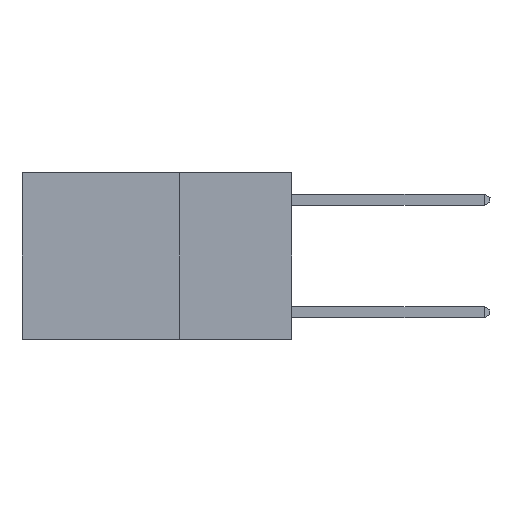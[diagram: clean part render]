
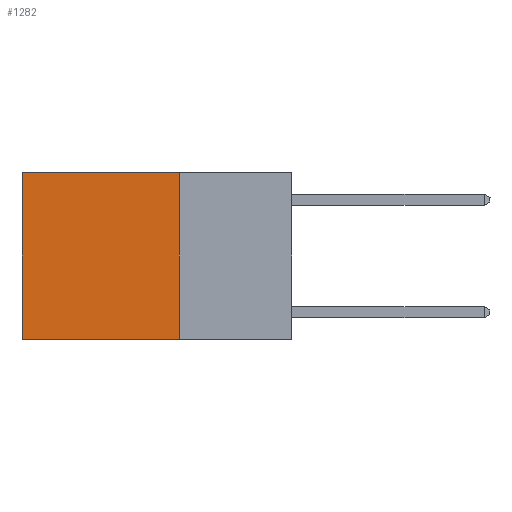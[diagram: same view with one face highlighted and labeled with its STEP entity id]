
A CAD part, left-side view. The second image highlights one B-rep face of the part: STEP entity #1282.
In plain terms, the highlighted planar face has unit normal (-1, 0, 0).
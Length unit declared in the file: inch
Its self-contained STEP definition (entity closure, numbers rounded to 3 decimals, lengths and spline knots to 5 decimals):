
#532 = ORIENTED_EDGE ( 'NONE', *, *, #2830, .F. ) ;
#539 = DIRECTION ( 'NONE',  ( 0., 1., 0. ) ) ;
#647 = EDGE_CURVE ( 'NONE', #7316, #4181, #1558, .T. ) ;
#650 = DIRECTION ( 'NONE',  ( 0., 0., -1. ) ) ;
#917 = DIRECTION ( 'NONE',  ( 0., 0., -1. ) ) ;
#1282 = ADVANCED_FACE ( 'NONE', ( #8568 ), #1535, .F. ) ;
#1535 = PLANE ( 'NONE',  #8107 ) ;
#1558 = LINE ( 'NONE', #3022, #9516 ) ;
#1604 = ORIENTED_EDGE ( 'NONE', *, *, #647, .T. ) ;
#1910 = CARTESIAN_POINT ( 'NONE',  ( 0.2625, 0.25, 0. ) ) ;
#2304 = EDGE_CURVE ( 'NONE', #7316, #6587, #8255, .T. ) ;
#2830 = EDGE_CURVE ( 'NONE', #6587, #6690, #4499, .T. ) ;
#3022 = CARTESIAN_POINT ( 'NONE',  ( 0.2625, 0.25, 0. ) ) ;
#3064 = LINE ( 'NONE', #4577, #8591 ) ;
#3335 = VECTOR ( 'NONE', #539, 39.37008 ) ;
#3782 = CARTESIAN_POINT ( 'NONE',  ( 0.2625, 0.25, -0.37 ) ) ;
#4181 = VERTEX_POINT ( 'NONE', #4224 ) ;
#4224 = CARTESIAN_POINT ( 'NONE',  ( 0.2625, 0.6, 0. ) ) ;
#4499 = LINE ( 'NONE', #3782, #3335 ) ;
#4577 = CARTESIAN_POINT ( 'NONE',  ( 0.2625, 0.6, 0. ) ) ;
#5544 = DIRECTION ( 'NONE',  ( 0., 1., 0. ) ) ;
#6587 = VERTEX_POINT ( 'NONE', #7937 ) ;
#6690 = VERTEX_POINT ( 'NONE', #7166 ) ;
#7166 = CARTESIAN_POINT ( 'NONE',  ( 0.2625, 0.6, -0.37 ) ) ;
#7316 = VERTEX_POINT ( 'NONE', #9916 ) ;
#7342 = ORIENTED_EDGE ( 'NONE', *, *, #2304, .F. ) ;
#7778 = CARTESIAN_POINT ( 'NONE',  ( 0.2625, 0.25, 0. ) ) ;
#7937 = CARTESIAN_POINT ( 'NONE',  ( 0.2625, 0.25, -0.37 ) ) ;
#8011 = VECTOR ( 'NONE', #917, 39.37008 ) ;
#8107 = AXIS2_PLACEMENT_3D ( 'NONE', #7778, #9532, #650 ) ;
#8132 = ORIENTED_EDGE ( 'NONE', *, *, #8236, .T. ) ;
#8236 = EDGE_CURVE ( 'NONE', #4181, #6690, #3064, .T. ) ;
#8255 = LINE ( 'NONE', #1910, #8011 ) ;
#8568 = FACE_OUTER_BOUND ( 'NONE', #9217, .T. ) ;
#8591 = VECTOR ( 'NONE', #10118, 39.37008 ) ;
#9217 = EDGE_LOOP ( 'NONE', ( #8132, #532, #7342, #1604 ) ) ;
#9516 = VECTOR ( 'NONE', #5544, 39.37008 ) ;
#9532 = DIRECTION ( 'NONE',  ( 1., 0., 0. ) ) ;
#9916 = CARTESIAN_POINT ( 'NONE',  ( 0.2625, 0.25, 0. ) ) ;
#10118 = DIRECTION ( 'NONE',  ( 0., 0., -1. ) ) ;
